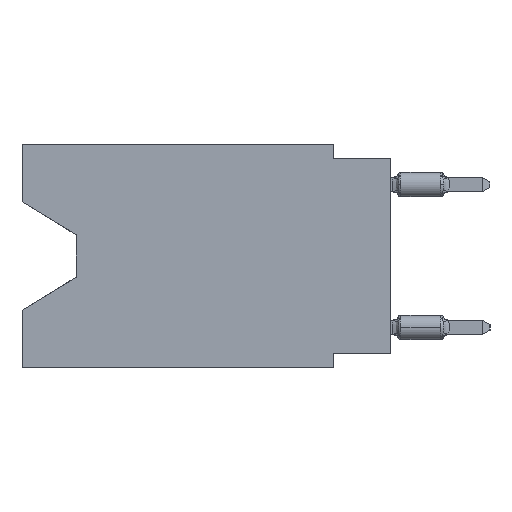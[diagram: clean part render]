
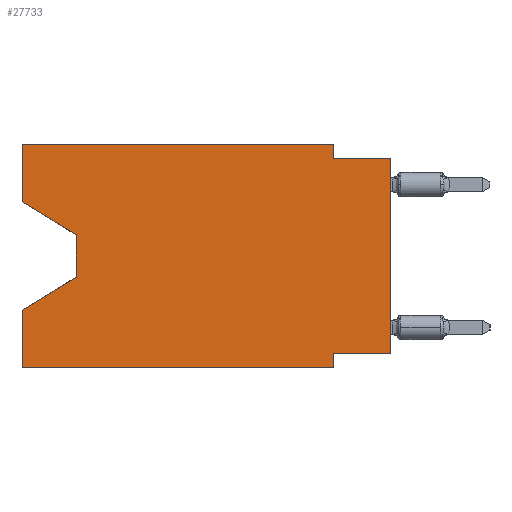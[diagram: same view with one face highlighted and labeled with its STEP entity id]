
A CAD part, left-side view. The second image highlights one B-rep face of the part: STEP entity #27733.
In plain terms, the highlighted planar face has unit normal (-1, 0, 0).
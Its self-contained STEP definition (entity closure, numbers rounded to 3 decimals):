
#225 = VECTOR ( 'NONE', #29321, 1000. ) ;
#293 = VECTOR ( 'NONE', #11369, 1000. ) ;
#699 = ORIENTED_EDGE ( 'NONE', *, *, #26365, .F. ) ;
#720 = VERTEX_POINT ( 'NONE', #24645 ) ;
#1008 = ORIENTED_EDGE ( 'NONE', *, *, #16076, .F. ) ;
#1135 = LINE ( 'NONE', #17561, #27895 ) ;
#1270 = LINE ( 'NONE', #17394, #26700 ) ;
#1427 = DIRECTION ( 'NONE',  ( 0., -1., 0. ) ) ;
#1854 = DIRECTION ( 'NONE',  ( 0., -0.855, -0.519 ) ) ;
#2220 = CARTESIAN_POINT ( 'NONE',  ( 0., 2.54, -9.271 ) ) ;
#2410 = CARTESIAN_POINT ( 'NONE',  ( 0., 16.383, 0. ) ) ;
#2842 = CARTESIAN_POINT ( 'NONE',  ( 0., 13.97, -5.893 ) ) ;
#3243 = ORIENTED_EDGE ( 'NONE', *, *, #4657, .F. ) ;
#3297 = ORIENTED_EDGE ( 'NONE', *, *, #10477, .F. ) ;
#3539 = VERTEX_POINT ( 'NONE', #29441 ) ;
#4657 = EDGE_CURVE ( 'NONE', #27417, #26939, #1135, .T. ) ;
#4693 = CARTESIAN_POINT ( 'NONE',  ( 0., 2.54, -9.906 ) ) ;
#5364 = ORIENTED_EDGE ( 'NONE', *, *, #20680, .T. ) ;
#5494 = DIRECTION ( 'NONE',  ( 0., 0., -1. ) ) ;
#6374 = LINE ( 'NONE', #10909, #18176 ) ;
#6708 = CARTESIAN_POINT ( 'NONE',  ( 0., 16.383, 0. ) ) ;
#6938 = VECTOR ( 'NONE', #5494, 1000. ) ;
#7259 = CARTESIAN_POINT ( 'NONE',  ( 0., 0., -0.635 ) ) ;
#7306 = FACE_OUTER_BOUND ( 'NONE', #13130, .T. ) ;
#7504 = VERTEX_POINT ( 'NONE', #19546 ) ;
#7856 = VERTEX_POINT ( 'NONE', #27959 ) ;
#8043 = LINE ( 'NONE', #14654, #12215 ) ;
#8981 = PLANE ( 'NONE',  #11817 ) ;
#9246 = DIRECTION ( 'NONE',  ( 0., 0., 1. ) ) ;
#9563 = VERTEX_POINT ( 'NONE', #2842 ) ;
#10477 = EDGE_CURVE ( 'NONE', #28776, #27417, #8043, .T. ) ;
#10684 = VERTEX_POINT ( 'NONE', #24881 ) ;
#10909 = CARTESIAN_POINT ( 'NONE',  ( 0., 16.383, -2.546 ) ) ;
#11192 = LINE ( 'NONE', #7259, #16054 ) ;
#11369 = DIRECTION ( 'NONE',  ( 0., 0., 1. ) ) ;
#11817 = AXIS2_PLACEMENT_3D ( 'NONE', #6708, #25103, #18170 ) ;
#11945 = CARTESIAN_POINT ( 'NONE',  ( 0., 16.383, 0. ) ) ;
#12127 = VERTEX_POINT ( 'NONE', #28356 ) ;
#12215 = VECTOR ( 'NONE', #28524, 1000. ) ;
#12414 = EDGE_CURVE ( 'NONE', #3539, #720, #23075, .T. ) ;
#12628 = DIRECTION ( 'NONE',  ( 0., 0., -1. ) ) ;
#12720 = CARTESIAN_POINT ( 'NONE',  ( 0., 13.97, -5.893 ) ) ;
#12782 = CARTESIAN_POINT ( 'NONE',  ( 0., 13.97, -4.013 ) ) ;
#13130 = EDGE_LOOP ( 'NONE', ( #19887, #24826, #18511, #15802, #21232, #3243, #3297, #5364, #22996, #699, #26174, #1008 ) ) ;
#13587 = DIRECTION ( 'NONE',  ( 0., -1., 0. ) ) ;
#13890 = LINE ( 'NONE', #23379, #21970 ) ;
#14654 = CARTESIAN_POINT ( 'NONE',  ( 0., 0., -9.271 ) ) ;
#14751 = CARTESIAN_POINT ( 'NONE',  ( 0., 16.383, -9.906 ) ) ;
#15802 = ORIENTED_EDGE ( 'NONE', *, *, #20123, .F. ) ;
#15872 = LINE ( 'NONE', #22666, #293 ) ;
#16054 = VECTOR ( 'NONE', #13587, 1000. ) ;
#16076 = EDGE_CURVE ( 'NONE', #12127, #3539, #25223, .T. ) ;
#16516 = EDGE_CURVE ( 'NONE', #7856, #10684, #11192, .T. ) ;
#16648 = VERTEX_POINT ( 'NONE', #14751 ) ;
#16672 = LINE ( 'NONE', #26150, #6938 ) ;
#17087 = VECTOR ( 'NONE', #27738, 1000. ) ;
#17394 = CARTESIAN_POINT ( 'NONE',  ( 0., 16.383, -9.906 ) ) ;
#17561 = CARTESIAN_POINT ( 'NONE',  ( 0., 2.54, -9.906 ) ) ;
#18170 = DIRECTION ( 'NONE',  ( 0., 0., -1. ) ) ;
#18176 = VECTOR ( 'NONE', #1854, 1000. ) ;
#18511 = ORIENTED_EDGE ( 'NONE', *, *, #25164, .T. ) ;
#19043 = EDGE_CURVE ( 'NONE', #21918, #9563, #24094, .T. ) ;
#19413 = VECTOR ( 'NONE', #9246, 1000. ) ;
#19546 = CARTESIAN_POINT ( 'NONE',  ( 0., 16.383, -7.36 ) ) ;
#19887 = ORIENTED_EDGE ( 'NONE', *, *, #29501, .T. ) ;
#20123 = EDGE_CURVE ( 'NONE', #16648, #7504, #15872, .T. ) ;
#20680 = EDGE_CURVE ( 'NONE', #28776, #10684, #13890, .T. ) ;
#21232 = ORIENTED_EDGE ( 'NONE', *, *, #25274, .T. ) ;
#21309 = CARTESIAN_POINT ( 'NONE',  ( 0., 13.97, -4.013 ) ) ;
#21918 = VERTEX_POINT ( 'NONE', #21309 ) ;
#21970 = VECTOR ( 'NONE', #23095, 1000. ) ;
#22455 = VECTOR ( 'NONE', #12628, 1000. ) ;
#22666 = CARTESIAN_POINT ( 'NONE',  ( 0., 16.383, 0. ) ) ;
#22996 = ORIENTED_EDGE ( 'NONE', *, *, #16516, .F. ) ;
#23075 = LINE ( 'NONE', #2410, #17087 ) ;
#23095 = DIRECTION ( 'NONE',  ( 0., 0., 1. ) ) ;
#23379 = CARTESIAN_POINT ( 'NONE',  ( 0., 0., 0. ) ) ;
#24094 = LINE ( 'NONE', #12782, #22455 ) ;
#24645 = CARTESIAN_POINT ( 'NONE',  ( 0., 2.54, 0. ) ) ;
#24826 = ORIENTED_EDGE ( 'NONE', *, *, #19043, .T. ) ;
#24881 = CARTESIAN_POINT ( 'NONE',  ( 0., 0., -0.635 ) ) ;
#25103 = DIRECTION ( 'NONE',  ( 1., 0., 0. ) ) ;
#25164 = EDGE_CURVE ( 'NONE', #9563, #7504, #29166, .T. ) ;
#25223 = LINE ( 'NONE', #11945, #19413 ) ;
#25274 = EDGE_CURVE ( 'NONE', #16648, #26939, #1270, .T. ) ;
#26150 = CARTESIAN_POINT ( 'NONE',  ( 0., 2.54, 0. ) ) ;
#26174 = ORIENTED_EDGE ( 'NONE', *, *, #12414, .F. ) ;
#26365 = EDGE_CURVE ( 'NONE', #720, #7856, #16672, .T. ) ;
#26700 = VECTOR ( 'NONE', #1427, 1000. ) ;
#26766 = DIRECTION ( 'NONE',  ( 0., 0., -1. ) ) ;
#26939 = VERTEX_POINT ( 'NONE', #4693 ) ;
#27092 = CARTESIAN_POINT ( 'NONE',  ( 0., 0., -9.271 ) ) ;
#27417 = VERTEX_POINT ( 'NONE', #2220 ) ;
#27733 = ADVANCED_FACE ( 'NONE', ( #7306 ), #8981, .F. ) ;
#27738 = DIRECTION ( 'NONE',  ( 0., -1., 0. ) ) ;
#27895 = VECTOR ( 'NONE', #26766, 1000. ) ;
#27959 = CARTESIAN_POINT ( 'NONE',  ( 0., 2.54, -0.635 ) ) ;
#28356 = CARTESIAN_POINT ( 'NONE',  ( 0., 16.383, -2.546 ) ) ;
#28524 = DIRECTION ( 'NONE',  ( 0., 1., 0. ) ) ;
#28776 = VERTEX_POINT ( 'NONE', #27092 ) ;
#29166 = LINE ( 'NONE', #12720, #225 ) ;
#29321 = DIRECTION ( 'NONE',  ( 0., 0.855, -0.519 ) ) ;
#29441 = CARTESIAN_POINT ( 'NONE',  ( 0., 16.383, 0. ) ) ;
#29501 = EDGE_CURVE ( 'NONE', #12127, #21918, #6374, .T. ) ;
